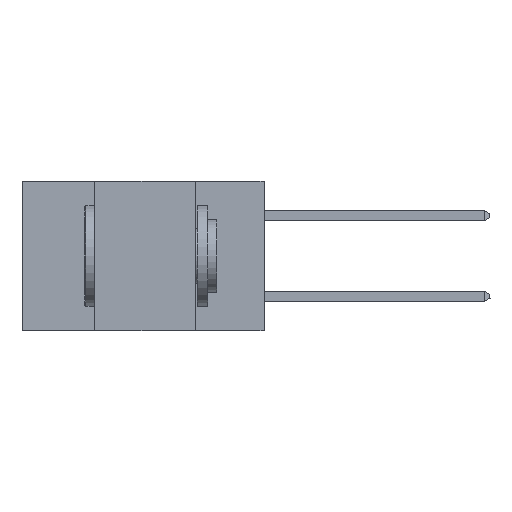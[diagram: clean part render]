
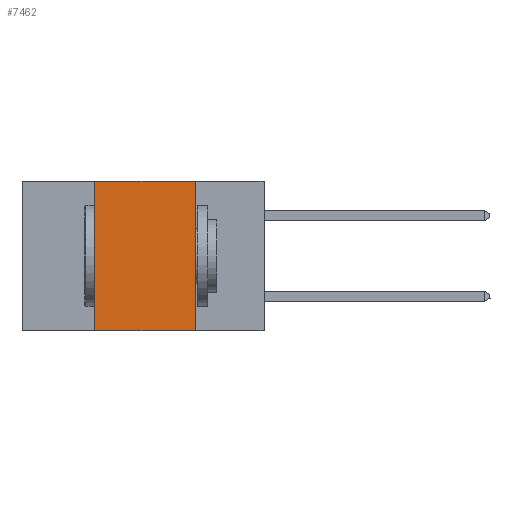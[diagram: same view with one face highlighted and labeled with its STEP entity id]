
A CAD part, left-side view. The second image highlights one B-rep face of the part: STEP entity #7462.
In plain terms, the highlighted planar face has unit normal (-1, 0, 0).
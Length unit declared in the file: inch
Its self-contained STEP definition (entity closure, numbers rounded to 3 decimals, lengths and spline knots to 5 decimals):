
#71 = VECTOR ( 'NONE', #6361, 39.37008 ) ;
#166 = VECTOR ( 'NONE', #323, 39.37008 ) ;
#323 = DIRECTION ( 'NONE',  ( 0., -1., 0. ) ) ;
#614 = CARTESIAN_POINT ( 'NONE',  ( 0., 0.42, 0. ) ) ;
#1612 = ORIENTED_EDGE ( 'NONE', *, *, #3995, .F. ) ;
#1803 = VECTOR ( 'NONE', #7643, 39.37008 ) ;
#2059 = CARTESIAN_POINT ( 'NONE',  ( 0., 0.6, 0. ) ) ;
#2062 = LINE ( 'NONE', #5492, #71 ) ;
#2546 = CARTESIAN_POINT ( 'NONE',  ( 0., 0.17, -0.37 ) ) ;
#2575 = VECTOR ( 'NONE', #8124, 39.37008 ) ;
#2611 = VERTEX_POINT ( 'NONE', #614 ) ;
#2944 = LINE ( 'NONE', #2059, #166 ) ;
#2987 = ORIENTED_EDGE ( 'NONE', *, *, #4490, .F. ) ;
#3090 = AXIS2_PLACEMENT_3D ( 'NONE', #9748, #6334, #8839 ) ;
#3262 = CARTESIAN_POINT ( 'NONE',  ( 0., 0.17, -0.37 ) ) ;
#3572 = ORIENTED_EDGE ( 'NONE', *, *, #4263, .T. ) ;
#3847 = PLANE ( 'NONE',  #3090 ) ;
#3995 = EDGE_CURVE ( 'NONE', #8265, #10291, #8316, .T. ) ;
#4229 = CARTESIAN_POINT ( 'NONE',  ( 0., 0.17, 0. ) ) ;
#4263 = EDGE_CURVE ( 'NONE', #6382, #10291, #5846, .T. ) ;
#4490 = EDGE_CURVE ( 'NONE', #6382, #2611, #2062, .T. ) ;
#5492 = CARTESIAN_POINT ( 'NONE',  ( 0., 0.42, -0.37 ) ) ;
#5846 = LINE ( 'NONE', #10313, #1803 ) ;
#6185 = EDGE_CURVE ( 'NONE', #2611, #8265, #2944, .T. ) ;
#6334 = DIRECTION ( 'NONE',  ( 1., 0., 0. ) ) ;
#6361 = DIRECTION ( 'NONE',  ( 0., 0., 1. ) ) ;
#6382 = VERTEX_POINT ( 'NONE', #7647 ) ;
#7462 = ADVANCED_FACE ( 'NONE', ( #9728 ), #3847, .F. ) ;
#7643 = DIRECTION ( 'NONE',  ( 0., -1., 0. ) ) ;
#7647 = CARTESIAN_POINT ( 'NONE',  ( 0., 0.42, -0.37 ) ) ;
#7677 = ORIENTED_EDGE ( 'NONE', *, *, #6185, .F. ) ;
#8124 = DIRECTION ( 'NONE',  ( 0., 0., -1. ) ) ;
#8265 = VERTEX_POINT ( 'NONE', #4229 ) ;
#8316 = LINE ( 'NONE', #3262, #2575 ) ;
#8839 = DIRECTION ( 'NONE',  ( 0., 0., -1. ) ) ;
#9728 = FACE_OUTER_BOUND ( 'NONE', #10194, .T. ) ;
#9748 = CARTESIAN_POINT ( 'NONE',  ( 0., 0.6, 0. ) ) ;
#10194 = EDGE_LOOP ( 'NONE', ( #1612, #7677, #2987, #3572 ) ) ;
#10291 = VERTEX_POINT ( 'NONE', #2546 ) ;
#10313 = CARTESIAN_POINT ( 'NONE',  ( 0., 0.6, -0.37 ) ) ;
